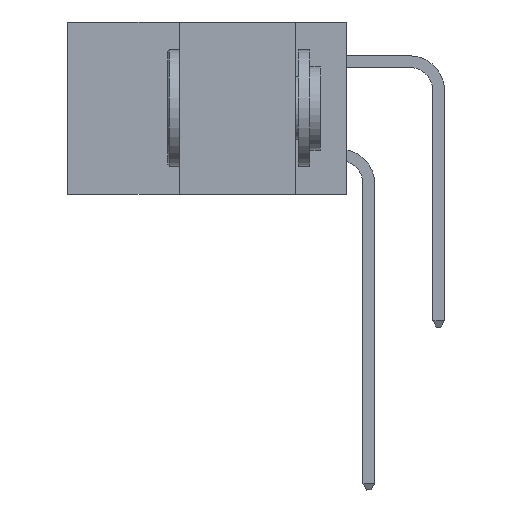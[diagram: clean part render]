
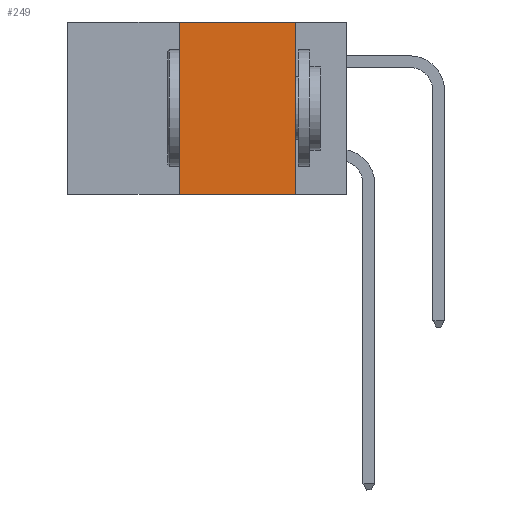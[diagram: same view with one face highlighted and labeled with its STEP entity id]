
A CAD part, left-side view. The second image highlights one B-rep face of the part: STEP entity #249.
In plain terms, the highlighted planar face has unit normal (-1, 0, 0).
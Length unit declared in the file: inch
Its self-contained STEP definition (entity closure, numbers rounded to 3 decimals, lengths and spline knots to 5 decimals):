
#153 = LINE ( 'NONE', #21612, #12013 ) ;
#249 = ADVANCED_FACE ( 'NONE', ( #19101 ), #5652, .F. ) ;
#356 = CARTESIAN_POINT ( 'NONE',  ( 0., 0.11, 0. ) ) ;
#685 = DIRECTION ( 'NONE',  ( 0., -1., 0. ) ) ;
#1787 = VERTEX_POINT ( 'NONE', #26563 ) ;
#2095 = CARTESIAN_POINT ( 'NONE',  ( 0., 0.6, 0. ) ) ;
#2991 = EDGE_CURVE ( 'NONE', #1787, #19323, #153, .T. ) ;
#3031 = EDGE_CURVE ( 'NONE', #8673, #27173, #11270, .T. ) ;
#3616 = CARTESIAN_POINT ( 'NONE',  ( 0., 0.36, -0.37 ) ) ;
#5580 = DIRECTION ( 'NONE',  ( 0., 0., -1. ) ) ;
#5608 = DIRECTION ( 'NONE',  ( 1., 0., 0. ) ) ;
#5652 = PLANE ( 'NONE',  #28619 ) ;
#8413 = ORIENTED_EDGE ( 'NONE', *, *, #3031, .T. ) ;
#8534 = VECTOR ( 'NONE', #11950, 39.37008 ) ;
#8673 = VERTEX_POINT ( 'NONE', #3616 ) ;
#9979 = DIRECTION ( 'NONE',  ( 0., -1., 0. ) ) ;
#11270 = LINE ( 'NONE', #21810, #22902 ) ;
#11455 = EDGE_LOOP ( 'NONE', ( #21180, #15372, #26598, #8413 ) ) ;
#11950 = DIRECTION ( 'NONE',  ( 0., 0., 1. ) ) ;
#12013 = VECTOR ( 'NONE', #9979, 39.37008 ) ;
#15372 = ORIENTED_EDGE ( 'NONE', *, *, #2991, .F. ) ;
#18796 = VECTOR ( 'NONE', #28335, 39.37008 ) ;
#19101 = FACE_OUTER_BOUND ( 'NONE', #11455, .T. ) ;
#19323 = VERTEX_POINT ( 'NONE', #29658 ) ;
#19497 = LINE ( 'NONE', #356, #18796 ) ;
#21180 = ORIENTED_EDGE ( 'NONE', *, *, #21920, .F. ) ;
#21186 = CARTESIAN_POINT ( 'NONE',  ( 0., 0.36, 0. ) ) ;
#21612 = CARTESIAN_POINT ( 'NONE',  ( 0., 0.6, 0. ) ) ;
#21810 = CARTESIAN_POINT ( 'NONE',  ( 0., 0.6, -0.37 ) ) ;
#21849 = EDGE_CURVE ( 'NONE', #8673, #1787, #27094, .T. ) ;
#21920 = EDGE_CURVE ( 'NONE', #19323, #27173, #19497, .T. ) ;
#22902 = VECTOR ( 'NONE', #685, 39.37008 ) ;
#26563 = CARTESIAN_POINT ( 'NONE',  ( 0., 0.36, 0. ) ) ;
#26598 = ORIENTED_EDGE ( 'NONE', *, *, #21849, .F. ) ;
#27094 = LINE ( 'NONE', #21186, #8534 ) ;
#27173 = VERTEX_POINT ( 'NONE', #28691 ) ;
#28335 = DIRECTION ( 'NONE',  ( 0., 0., -1. ) ) ;
#28619 = AXIS2_PLACEMENT_3D ( 'NONE', #2095, #5608, #5580 ) ;
#28691 = CARTESIAN_POINT ( 'NONE',  ( 0., 0.11, -0.37 ) ) ;
#29658 = CARTESIAN_POINT ( 'NONE',  ( 0., 0.11, 0. ) ) ;
